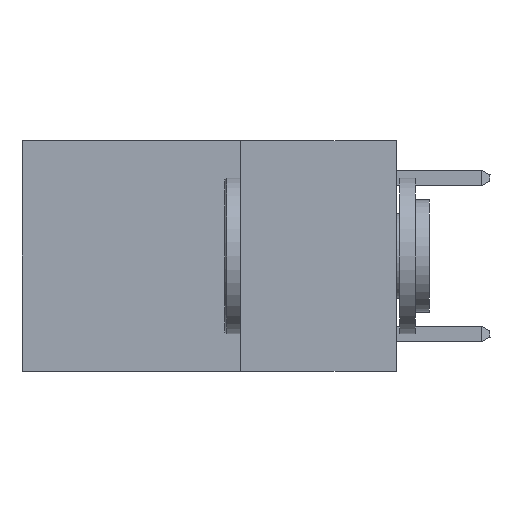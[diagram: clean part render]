
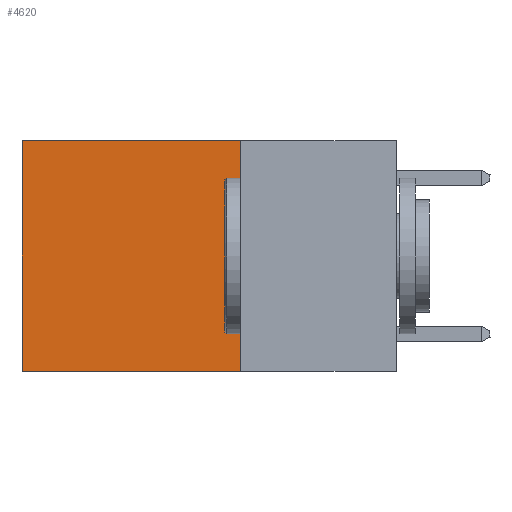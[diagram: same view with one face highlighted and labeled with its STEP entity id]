
A CAD part, left-side view. The second image highlights one B-rep face of the part: STEP entity #4620.
In plain terms, the highlighted planar face has unit normal (-1, 0, 0).
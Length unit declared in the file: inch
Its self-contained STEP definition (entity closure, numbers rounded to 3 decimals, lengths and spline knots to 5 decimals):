
#193 = LINE ( 'NONE', #5649, #7763 ) ;
#614 = CARTESIAN_POINT ( 'NONE',  ( 0.2625, 0.25, -0.37 ) ) ;
#640 = CARTESIAN_POINT ( 'NONE',  ( 0.2625, 0.25, -0.37 ) ) ;
#925 = DIRECTION ( 'NONE',  ( 0., 1., 0. ) ) ;
#1455 = EDGE_CURVE ( 'NONE', #10918, #2723, #11296, .T. ) ;
#2062 = ORIENTED_EDGE ( 'NONE', *, *, #9301, .T. ) ;
#2380 = VECTOR ( 'NONE', #925, 39.37008 ) ;
#2723 = VERTEX_POINT ( 'NONE', #6861 ) ;
#2878 = LINE ( 'NONE', #5676, #8841 ) ;
#4620 = ADVANCED_FACE ( 'NONE', ( #11576 ), #9578, .F. ) ;
#4865 = EDGE_CURVE ( 'NONE', #10918, #9608, #193, .T. ) ;
#4929 = DIRECTION ( 'NONE',  ( 0., 0., -1. ) ) ;
#5070 = AXIS2_PLACEMENT_3D ( 'NONE', #9798, #10548, #4929 ) ;
#5155 = EDGE_CURVE ( 'NONE', #9608, #5307, #6128, .T. ) ;
#5307 = VERTEX_POINT ( 'NONE', #5872 ) ;
#5529 = DIRECTION ( 'NONE',  ( 0., 0., -1. ) ) ;
#5649 = CARTESIAN_POINT ( 'NONE',  ( 0.2625, 0.25, 0. ) ) ;
#5676 = CARTESIAN_POINT ( 'NONE',  ( 0.2625, 0.6, 0. ) ) ;
#5872 = CARTESIAN_POINT ( 'NONE',  ( 0.2625, 0.6, -0.37 ) ) ;
#6128 = LINE ( 'NONE', #614, #2380 ) ;
#6386 = ORIENTED_EDGE ( 'NONE', *, *, #1455, .T. ) ;
#6581 = EDGE_LOOP ( 'NONE', ( #2062, #6702, #7197, #6386 ) ) ;
#6702 = ORIENTED_EDGE ( 'NONE', *, *, #5155, .F. ) ;
#6861 = CARTESIAN_POINT ( 'NONE',  ( 0.2625, 0.6, 0. ) ) ;
#7197 = ORIENTED_EDGE ( 'NONE', *, *, #4865, .F. ) ;
#7763 = VECTOR ( 'NONE', #5529, 39.37008 ) ;
#8262 = DIRECTION ( 'NONE',  ( 0., 0., -1. ) ) ;
#8841 = VECTOR ( 'NONE', #8262, 39.37008 ) ;
#9301 = EDGE_CURVE ( 'NONE', #2723, #5307, #2878, .T. ) ;
#9578 = PLANE ( 'NONE',  #5070 ) ;
#9608 = VERTEX_POINT ( 'NONE', #640 ) ;
#9798 = CARTESIAN_POINT ( 'NONE',  ( 0.2625, 0.25, 0. ) ) ;
#9955 = VECTOR ( 'NONE', #11357, 39.37008 ) ;
#10380 = CARTESIAN_POINT ( 'NONE',  ( 0.2625, 0.25, 0. ) ) ;
#10548 = DIRECTION ( 'NONE',  ( 1., 0., 0. ) ) ;
#10876 = CARTESIAN_POINT ( 'NONE',  ( 0.2625, 0.25, 0. ) ) ;
#10918 = VERTEX_POINT ( 'NONE', #10876 ) ;
#11296 = LINE ( 'NONE', #10380, #9955 ) ;
#11357 = DIRECTION ( 'NONE',  ( 0., 1., 0. ) ) ;
#11576 = FACE_OUTER_BOUND ( 'NONE', #6581, .T. ) ;
